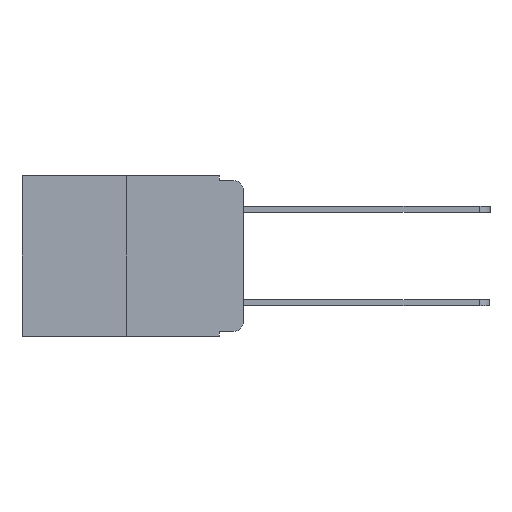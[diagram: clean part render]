
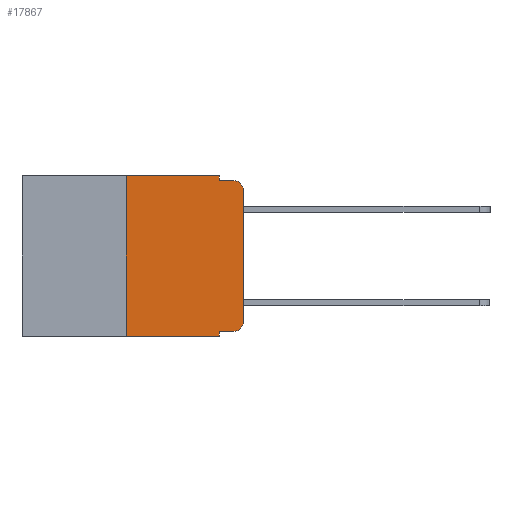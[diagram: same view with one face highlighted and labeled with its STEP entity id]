
A CAD part, left-side view. The second image highlights one B-rep face of the part: STEP entity #17867.
In plain terms, the highlighted planar face has unit normal (-1, 0, 0).
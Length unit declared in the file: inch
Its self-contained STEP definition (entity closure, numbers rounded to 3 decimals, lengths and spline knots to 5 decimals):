
#136 = ORIENTED_EDGE ( 'NONE', *, *, #9085, .F. ) ;
#211 = DIRECTION ( 'NONE',  ( -1., 0., 0. ) ) ;
#555 = CARTESIAN_POINT ( 'NONE',  ( 0., 0.473, 0. ) ) ;
#1368 = EDGE_CURVE ( 'NONE', #3269, #18000, #5052, .T. ) ;
#1573 = ORIENTED_EDGE ( 'NONE', *, *, #7169, .F. ) ;
#1608 = CARTESIAN_POINT ( 'NONE',  ( 0., 0., -0.313 ) ) ;
#1771 = VECTOR ( 'NONE', #16220, 39.37008 ) ;
#2029 = ORIENTED_EDGE ( 'NONE', *, *, #18184, .T. ) ;
#2213 = CARTESIAN_POINT ( 'NONE',  ( 0., 0.02, -0.01 ) ) ;
#2334 = CARTESIAN_POINT ( 'NONE',  ( 0., 0.051, 0. ) ) ;
#2404 = VERTEX_POINT ( 'NONE', #2874 ) ;
#2544 = ORIENTED_EDGE ( 'NONE', *, *, #3352, .T. ) ;
#2812 = AXIS2_PLACEMENT_3D ( 'NONE', #13967, #4226, #14027 ) ;
#2830 = ORIENTED_EDGE ( 'NONE', *, *, #1368, .T. ) ;
#2874 = CARTESIAN_POINT ( 'NONE',  ( 0., 0.25, -0.343 ) ) ;
#2974 = VECTOR ( 'NONE', #5207, 39.37008 ) ;
#3062 = VECTOR ( 'NONE', #14669, 39.37008 ) ;
#3070 = ORIENTED_EDGE ( 'NONE', *, *, #15532, .T. ) ;
#3269 = VERTEX_POINT ( 'NONE', #9633 ) ;
#3352 = EDGE_CURVE ( 'NONE', #14368, #3269, #17746, .T. ) ;
#3491 = VERTEX_POINT ( 'NONE', #8361 ) ;
#4226 = DIRECTION ( 'NONE',  ( 1., 0., 0. ) ) ;
#4557 = ORIENTED_EDGE ( 'NONE', *, *, #14620, .F. ) ;
#4644 = EDGE_LOOP ( 'NONE', ( #2029, #3070, #4557, #5963, #7417, #136, #7966, #1573, #2544, #2830 ) ) ;
#5052 = CIRCLE ( 'NONE', #13893, 0.02 ) ;
#5073 = FACE_OUTER_BOUND ( 'NONE', #4644, .T. ) ;
#5207 = DIRECTION ( 'NONE',  ( 0., 0., -1. ) ) ;
#5674 = LINE ( 'NONE', #17547, #9016 ) ;
#5963 = ORIENTED_EDGE ( 'NONE', *, *, #12796, .F. ) ;
#5994 = AXIS2_PLACEMENT_3D ( 'NONE', #8876, #211, #10294 ) ;
#6303 = LINE ( 'NONE', #7840, #10083 ) ;
#6309 = CARTESIAN_POINT ( 'NONE',  ( 0., 0., 0. ) ) ;
#6490 = VECTOR ( 'NONE', #15390, 39.37008 ) ;
#6719 = VERTEX_POINT ( 'NONE', #16683 ) ;
#6724 = CARTESIAN_POINT ( 'NONE',  ( 0., 0.02, -0.313 ) ) ;
#6728 = CIRCLE ( 'NONE', #5994, 0.02 ) ;
#7070 = CARTESIAN_POINT ( 'NONE',  ( 0., 0.25, 0. ) ) ;
#7169 = EDGE_CURVE ( 'NONE', #14368, #12834, #13754, .T. ) ;
#7417 = ORIENTED_EDGE ( 'NONE', *, *, #10727, .F. ) ;
#7840 = CARTESIAN_POINT ( 'NONE',  ( 0., 0.051, -0.01 ) ) ;
#7956 = CARTESIAN_POINT ( 'NONE',  ( 0., 0.473, -0.343 ) ) ;
#7966 = ORIENTED_EDGE ( 'NONE', *, *, #15757, .T. ) ;
#8361 = CARTESIAN_POINT ( 'NONE',  ( 0., 0.051, 0. ) ) ;
#8645 = CARTESIAN_POINT ( 'NONE',  ( 0., 0.051, -0.333 ) ) ;
#8876 = CARTESIAN_POINT ( 'NONE',  ( 0., 0.02, -0.03 ) ) ;
#8931 = LINE ( 'NONE', #7070, #6490 ) ;
#8933 = LINE ( 'NONE', #7956, #1771 ) ;
#8935 = CARTESIAN_POINT ( 'NONE',  ( 0., 0.051, -0.333 ) ) ;
#9016 = VECTOR ( 'NONE', #9404, 39.37008 ) ;
#9085 = EDGE_CURVE ( 'NONE', #2404, #17410, #8931, .T. ) ;
#9320 = VECTOR ( 'NONE', #17493, 39.37008 ) ;
#9404 = DIRECTION ( 'NONE',  ( 0., 0., -1. ) ) ;
#9633 = CARTESIAN_POINT ( 'NONE',  ( 0., 0.02, -0.333 ) ) ;
#10083 = VECTOR ( 'NONE', #16113, 39.37008 ) ;
#10294 = DIRECTION ( 'NONE',  ( 0., 0., -1. ) ) ;
#10727 = EDGE_CURVE ( 'NONE', #17410, #3491, #16596, .T. ) ;
#10858 = CARTESIAN_POINT ( 'NONE',  ( 0., 0.051, -0.01 ) ) ;
#12342 = DIRECTION ( 'NONE',  ( -1., 0., 0. ) ) ;
#12662 = PLANE ( 'NONE',  #2812 ) ;
#12796 = EDGE_CURVE ( 'NONE', #3491, #17013, #5674, .T. ) ;
#12834 = VERTEX_POINT ( 'NONE', #17604 ) ;
#13078 = DIRECTION ( 'NONE',  ( 0., 0., -1. ) ) ;
#13754 = LINE ( 'NONE', #2334, #2974 ) ;
#13893 = AXIS2_PLACEMENT_3D ( 'NONE', #6724, #12342, #13078 ) ;
#13967 = CARTESIAN_POINT ( 'NONE',  ( 0., 0.473, 0. ) ) ;
#14027 = DIRECTION ( 'NONE',  ( 0., 0., -1. ) ) ;
#14187 = VECTOR ( 'NONE', #17713, 39.37008 ) ;
#14368 = VERTEX_POINT ( 'NONE', #8645 ) ;
#14620 = EDGE_CURVE ( 'NONE', #17013, #16967, #6303, .T. ) ;
#14669 = DIRECTION ( 'NONE',  ( 0., 0., 1. ) ) ;
#15390 = DIRECTION ( 'NONE',  ( 0., 0., 1. ) ) ;
#15532 = EDGE_CURVE ( 'NONE', #6719, #16967, #6728, .T. ) ;
#15757 = EDGE_CURVE ( 'NONE', #2404, #12834, #8933, .T. ) ;
#16113 = DIRECTION ( 'NONE',  ( 0., -1., 0. ) ) ;
#16160 = CARTESIAN_POINT ( 'NONE',  ( 0., 0.25, 0. ) ) ;
#16220 = DIRECTION ( 'NONE',  ( 0., -1., 0. ) ) ;
#16596 = LINE ( 'NONE', #555, #9320 ) ;
#16683 = CARTESIAN_POINT ( 'NONE',  ( 0., 0., -0.03 ) ) ;
#16967 = VERTEX_POINT ( 'NONE', #2213 ) ;
#17013 = VERTEX_POINT ( 'NONE', #10858 ) ;
#17410 = VERTEX_POINT ( 'NONE', #16160 ) ;
#17493 = DIRECTION ( 'NONE',  ( 0., -1., 0. ) ) ;
#17547 = CARTESIAN_POINT ( 'NONE',  ( 0., 0.051, 0. ) ) ;
#17604 = CARTESIAN_POINT ( 'NONE',  ( 0., 0.051, -0.343 ) ) ;
#17713 = DIRECTION ( 'NONE',  ( 0., -1., 0. ) ) ;
#17746 = LINE ( 'NONE', #8935, #14187 ) ;
#17793 = LINE ( 'NONE', #6309, #3062 ) ;
#17867 = ADVANCED_FACE ( 'NONE', ( #5073 ), #12662, .F. ) ;
#18000 = VERTEX_POINT ( 'NONE', #1608 ) ;
#18184 = EDGE_CURVE ( 'NONE', #18000, #6719, #17793, .T. ) ;
